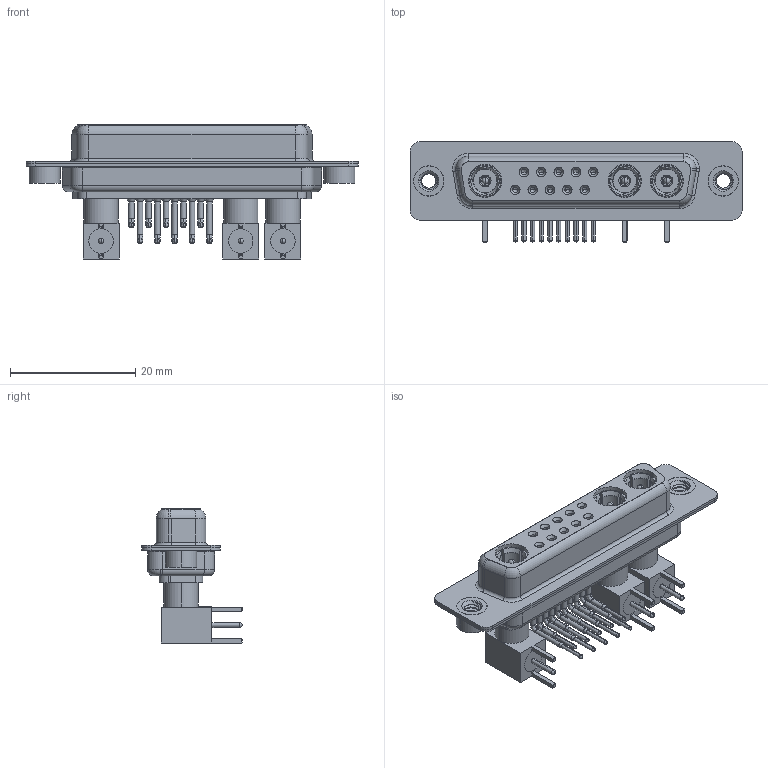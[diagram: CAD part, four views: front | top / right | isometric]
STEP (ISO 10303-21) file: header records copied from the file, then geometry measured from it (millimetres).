
FILE_DESCRIPTION (( 'STEP AP203' ), '1' );
FILE_NAME ('630-13W3640-7N2.STEP', '2022-06-01T18:06:18', ( '' ), ( '' ), 'SwSTEP 2.0', 'SolidWorks 2020', '' );
FILE_SCHEMA (( 'CONFIG_CONTROL_DESIGN' ));
Length unit declared in the file: millimetre
Products named in the file (16): 630-13W3640-7N2; Co-Ax Plug_RA PC Tail; Locking Collar; RA Back Shell; Insulator RA Pin; 630Combo Contact Row 2; Insulator Pin_Straight PC Tail; 630Combo Shell Front_25 Contacts; Co-Ax Plug Assy_RA; Pin_RA; 630Combo Contact Row 1; 630Combo Shell Rear_25 Contacts; 630Combo Threaded Rivet_2; 630Combo Housing_13W3
Assembly tree (36 placements, depth 3):
  630-13W3640-7N2
    630Combo Housing_13W3
    630Combo Shell Front_25 Contacts
    630Combo Shell Rear_25 Contacts
    630Combo Threaded Rivet_2  x2
    Co-Ax Plug Assy_RA
      Co-Ax Plug_RA PC Tail
      Insulator Pin_Straight PC Tail
      Pin_RA
      Locking Collar
      RA Back Shell
      Insulator RA Pin
    Co-Ax Plug Assy_RA
      Co-Ax Plug_RA PC Tail
      Insulator Pin_Straight PC Tail
      Pin_RA
      Locking Collar
      RA Back Shell
      Insulator RA Pin
    Co-Ax Plug Assy_RA
      Co-Ax Plug_RA PC Tail
      Insulator Pin_Straight PC Tail
      Pin_RA
      Locking Collar
      RA Back Shell
      Insulator RA Pin
    630Combo Contact Row 1  x5
    630Combo Contact Row 2  x5
Bounding box: 53.05 x 16 x 21.41 mm (x, y, z)
Volume: 4523.1 mm3; surface area: 10883.7 mm2
Topology: 33 solids, 33 shells, 1313 faces, 3238 edges, 2030 vertices
Faces by surface type: cylinder 562, plane 418, cone 197, torus 75, bspline 49, sphere 12
Entity records: 22697 total; most frequent: CARTESIAN_POINT 5201, DIRECTION 3470, ORIENTED_EDGE 3006, EDGE_CURVE 1503, AXIS2_PLACEMENT_3D 1422, VERTEX_POINT 954, CIRCLE 758, EDGE_LOOP 743
